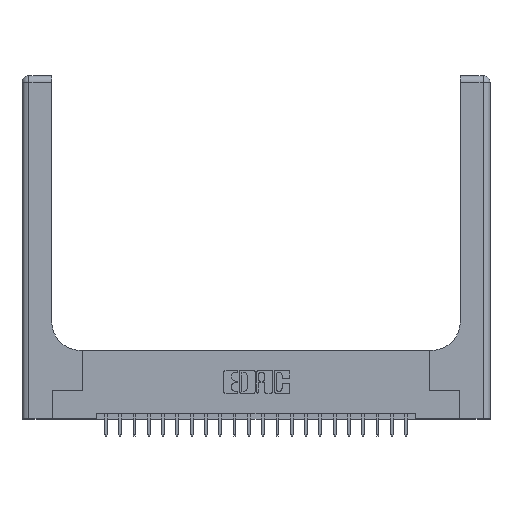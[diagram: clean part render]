
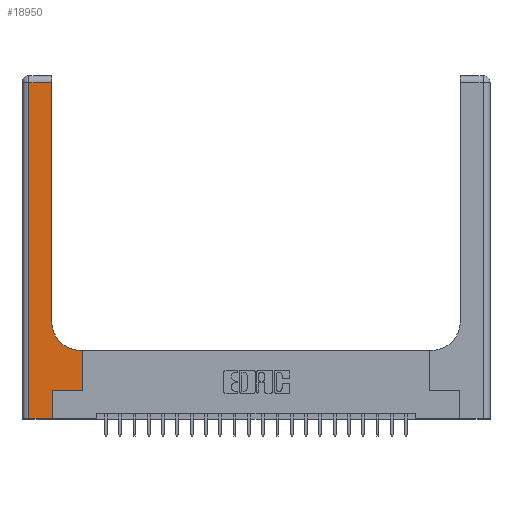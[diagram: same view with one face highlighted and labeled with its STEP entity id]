
A CAD part, top view. The second image highlights one B-rep face of the part: STEP entity #18950.
In plain terms, the highlighted planar face has unit normal (0, 0, 1).
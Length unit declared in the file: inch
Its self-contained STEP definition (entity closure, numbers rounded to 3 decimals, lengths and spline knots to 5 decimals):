
#84 = VERTEX_POINT ( 'NONE', #2844 ) ;
#668 = LINE ( 'NONE', #11224, #10079 ) ;
#894 = CARTESIAN_POINT ( 'NONE',  ( 0.06, 3., 0.37 ) ) ;
#1446 = CIRCLE ( 'NONE', #2182, 0.25 ) ;
#1514 = VECTOR ( 'NONE', #11883, 39.37008 ) ;
#1673 = CARTESIAN_POINT ( 'NONE',  ( 0.26, 0.6, 0.37 ) ) ;
#1806 = DIRECTION ( 'NONE',  ( -1., 0., 0. ) ) ;
#1953 = LINE ( 'NONE', #8947, #14738 ) ;
#2182 = AXIS2_PLACEMENT_3D ( 'NONE', #21780, #18674, #13028 ) ;
#2615 = LINE ( 'NONE', #894, #13710 ) ;
#2844 = CARTESIAN_POINT ( 'NONE',  ( 0.06, 0., 0.37 ) ) ;
#3185 = CARTESIAN_POINT ( 'NONE',  ( 0., 2.94, 0.37 ) ) ;
#3297 = CARTESIAN_POINT ( 'NONE',  ( 0.06, 2.94, 0.37 ) ) ;
#3305 = DIRECTION ( 'NONE',  ( 0., 0., -1. ) ) ;
#3742 = VECTOR ( 'NONE', #10841, 39.37008 ) ;
#3790 = CARTESIAN_POINT ( 'NONE',  ( 0.26, 2.94, 0.37 ) ) ;
#3938 = VERTEX_POINT ( 'NONE', #3297 ) ;
#4165 = EDGE_CURVE ( 'NONE', #12992, #10143, #1446, .T. ) ;
#4542 = VERTEX_POINT ( 'NONE', #16538 ) ;
#5006 = DIRECTION ( 'NONE',  ( 0., 1., 0. ) ) ;
#5597 = VECTOR ( 'NONE', #5006, 39.37008 ) ;
#6245 = VECTOR ( 'NONE', #10170, 39.37008 ) ;
#7064 = LINE ( 'NONE', #15414, #5597 ) ;
#7660 = ORIENTED_EDGE ( 'NONE', *, *, #4165, .T. ) ;
#7787 = DIRECTION ( 'NONE',  ( 0., -1., 0. ) ) ;
#8360 = FACE_OUTER_BOUND ( 'NONE', #13602, .T. ) ;
#8474 = PLANE ( 'NONE',  #21749 ) ;
#8784 = EDGE_CURVE ( 'NONE', #22053, #14337, #1953, .T. ) ;
#8947 = CARTESIAN_POINT ( 'NONE',  ( 0.265, 0.25, 0.37 ) ) ;
#9120 = LINE ( 'NONE', #16096, #3742 ) ;
#9485 = LINE ( 'NONE', #16817, #22033 ) ;
#9502 = DIRECTION ( 'NONE',  ( 0., 1., 0. ) ) ;
#9573 = ORIENTED_EDGE ( 'NONE', *, *, #15835, .T. ) ;
#9871 = CARTESIAN_POINT ( 'NONE',  ( 0.528, 0.25, 0.37 ) ) ;
#9952 = VERTEX_POINT ( 'NONE', #3790 ) ;
#10079 = VECTOR ( 'NONE', #9502, 39.37008 ) ;
#10143 = VERTEX_POINT ( 'NONE', #11916 ) ;
#10170 = DIRECTION ( 'NONE',  ( -1., 0., 0. ) ) ;
#10427 = EDGE_CURVE ( 'NONE', #3938, #84, #2615, .T. ) ;
#10841 = DIRECTION ( 'NONE',  ( 0., 1., 0. ) ) ;
#11140 = CARTESIAN_POINT ( 'NONE',  ( 0.51, 0.6, 0.37 ) ) ;
#11201 = VERTEX_POINT ( 'NONE', #16071 ) ;
#11224 = CARTESIAN_POINT ( 'NONE',  ( 0.26, 3., 0.37 ) ) ;
#11741 = EDGE_CURVE ( 'NONE', #10143, #9952, #668, .T. ) ;
#11883 = DIRECTION ( 'NONE',  ( -1., 0., 0. ) ) ;
#11916 = CARTESIAN_POINT ( 'NONE',  ( 0.26, 0.85, 0.37 ) ) ;
#12580 = ORIENTED_EDGE ( 'NONE', *, *, #10427, .T. ) ;
#12751 = ORIENTED_EDGE ( 'NONE', *, *, #17260, .T. ) ;
#12992 = VERTEX_POINT ( 'NONE', #11140 ) ;
#13028 = DIRECTION ( 'NONE',  ( 1., 0., 0. ) ) ;
#13399 = ORIENTED_EDGE ( 'NONE', *, *, #18424, .T. ) ;
#13597 = LINE ( 'NONE', #1673, #1514 ) ;
#13602 = EDGE_LOOP ( 'NONE', ( #19676, #13399, #12580, #9573, #20337, #21705, #12751, #22057, #7660 ) ) ;
#13710 = VECTOR ( 'NONE', #7787, 39.37008 ) ;
#14337 = VERTEX_POINT ( 'NONE', #9871 ) ;
#14738 = VECTOR ( 'NONE', #15919, 39.37008 ) ;
#14974 = DIRECTION ( 'NONE',  ( 1., 0., 0. ) ) ;
#15414 = CARTESIAN_POINT ( 'NONE',  ( 0.265, 0., 0.37 ) ) ;
#15835 = EDGE_CURVE ( 'NONE', #84, #11201, #9485, .T. ) ;
#15919 = DIRECTION ( 'NONE',  ( 1., 0., 0. ) ) ;
#16071 = CARTESIAN_POINT ( 'NONE',  ( 0.265, 0., 0.37 ) ) ;
#16096 = CARTESIAN_POINT ( 'NONE',  ( 0.528, 0.25, 0.37 ) ) ;
#16538 = CARTESIAN_POINT ( 'NONE',  ( 0.528, 0.6, 0.37 ) ) ;
#16817 = CARTESIAN_POINT ( 'NONE',  ( 0., 0., 0.37 ) ) ;
#17260 = EDGE_CURVE ( 'NONE', #14337, #4542, #9120, .T. ) ;
#18424 = EDGE_CURVE ( 'NONE', #9952, #3938, #18923, .T. ) ;
#18659 = CARTESIAN_POINT ( 'NONE',  ( 0.265, 0.25, 0.37 ) ) ;
#18674 = DIRECTION ( 'NONE',  ( 0., 0., -1. ) ) ;
#18923 = LINE ( 'NONE', #3185, #6245 ) ;
#18950 = ADVANCED_FACE ( 'NONE', ( #8360 ), #8474, .F. ) ;
#19040 = CARTESIAN_POINT ( 'NONE',  ( 0., 3., 0.37 ) ) ;
#19676 = ORIENTED_EDGE ( 'NONE', *, *, #11741, .T. ) ;
#20337 = ORIENTED_EDGE ( 'NONE', *, *, #21839, .T. ) ;
#20590 = EDGE_CURVE ( 'NONE', #4542, #12992, #13597, .T. ) ;
#21705 = ORIENTED_EDGE ( 'NONE', *, *, #8784, .T. ) ;
#21749 = AXIS2_PLACEMENT_3D ( 'NONE', #19040, #3305, #1806 ) ;
#21780 = CARTESIAN_POINT ( 'NONE',  ( 0.51, 0.85, 0.37 ) ) ;
#21839 = EDGE_CURVE ( 'NONE', #11201, #22053, #7064, .T. ) ;
#22033 = VECTOR ( 'NONE', #14974, 39.37008 ) ;
#22053 = VERTEX_POINT ( 'NONE', #18659 ) ;
#22057 = ORIENTED_EDGE ( 'NONE', *, *, #20590, .T. ) ;
